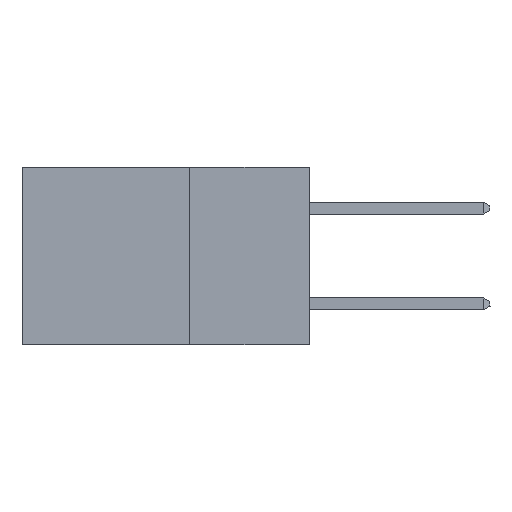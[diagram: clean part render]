
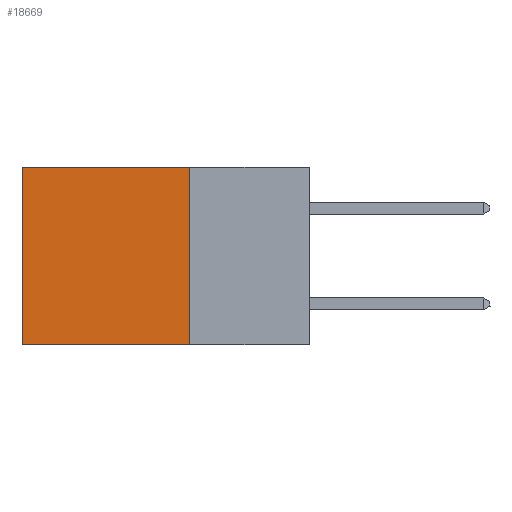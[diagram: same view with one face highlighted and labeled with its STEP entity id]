
A CAD part, left-side view. The second image highlights one B-rep face of the part: STEP entity #18669.
In plain terms, the highlighted planar face has unit normal (-1, 0, 0).
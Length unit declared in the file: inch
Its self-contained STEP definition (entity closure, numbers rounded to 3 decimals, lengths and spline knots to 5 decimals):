
#2046 = DIRECTION ( 'NONE',  ( 0., 0., -1. ) ) ;
#2988 = CARTESIAN_POINT ( 'NONE',  ( 0.2875, 0.25, -0.37 ) ) ;
#3006 = DIRECTION ( 'NONE',  ( 0., 1., 0. ) ) ;
#4272 = LINE ( 'NONE', #16524, #14862 ) ;
#4389 = CARTESIAN_POINT ( 'NONE',  ( 0.2875, 0.25, 0. ) ) ;
#4454 = VERTEX_POINT ( 'NONE', #2988 ) ;
#4736 = CARTESIAN_POINT ( 'NONE',  ( 0.2875, 0.25, 0. ) ) ;
#6127 = DIRECTION ( 'NONE',  ( 0., 1., 0. ) ) ;
#6477 = DIRECTION ( 'NONE',  ( 0., 0., -1. ) ) ;
#6876 = LINE ( 'NONE', #12257, #11846 ) ;
#7324 = ORIENTED_EDGE ( 'NONE', *, *, #10382, .F. ) ;
#7426 = VERTEX_POINT ( 'NONE', #8928 ) ;
#8843 = EDGE_CURVE ( 'NONE', #9002, #20833, #4272, .T. ) ;
#8928 = CARTESIAN_POINT ( 'NONE',  ( 0.2875, 0.25, 0. ) ) ;
#8973 = LINE ( 'NONE', #4389, #21231 ) ;
#9002 = VERTEX_POINT ( 'NONE', #11857 ) ;
#10236 = LINE ( 'NONE', #13157, #14783 ) ;
#10382 = EDGE_CURVE ( 'NONE', #7426, #4454, #6876, .T. ) ;
#11126 = ORIENTED_EDGE ( 'NONE', *, *, #20365, .T. ) ;
#11583 = FACE_OUTER_BOUND ( 'NONE', #12918, .T. ) ;
#11846 = VECTOR ( 'NONE', #2046, 39.37008 ) ;
#11857 = CARTESIAN_POINT ( 'NONE',  ( 0.2875, 0.6, 0. ) ) ;
#12257 = CARTESIAN_POINT ( 'NONE',  ( 0.2875, 0.25, 0. ) ) ;
#12918 = EDGE_LOOP ( 'NONE', ( #19406, #12992, #7324, #11126 ) ) ;
#12992 = ORIENTED_EDGE ( 'NONE', *, *, #20486, .F. ) ;
#13157 = CARTESIAN_POINT ( 'NONE',  ( 0.2875, 0.25, -0.37 ) ) ;
#14783 = VECTOR ( 'NONE', #3006, 39.37008 ) ;
#14862 = VECTOR ( 'NONE', #19831, 39.37008 ) ;
#16524 = CARTESIAN_POINT ( 'NONE',  ( 0.2875, 0.6, 0. ) ) ;
#16553 = DIRECTION ( 'NONE',  ( 1., 0., 0. ) ) ;
#16700 = CARTESIAN_POINT ( 'NONE',  ( 0.2875, 0.6, -0.37 ) ) ;
#18142 = PLANE ( 'NONE',  #19423 ) ;
#18669 = ADVANCED_FACE ( 'NONE', ( #11583 ), #18142, .F. ) ;
#19406 = ORIENTED_EDGE ( 'NONE', *, *, #8843, .T. ) ;
#19423 = AXIS2_PLACEMENT_3D ( 'NONE', #4736, #16553, #6477 ) ;
#19831 = DIRECTION ( 'NONE',  ( 0., 0., -1. ) ) ;
#20365 = EDGE_CURVE ( 'NONE', #7426, #9002, #8973, .T. ) ;
#20486 = EDGE_CURVE ( 'NONE', #4454, #20833, #10236, .T. ) ;
#20833 = VERTEX_POINT ( 'NONE', #16700 ) ;
#21231 = VECTOR ( 'NONE', #6127, 39.37008 ) ;
